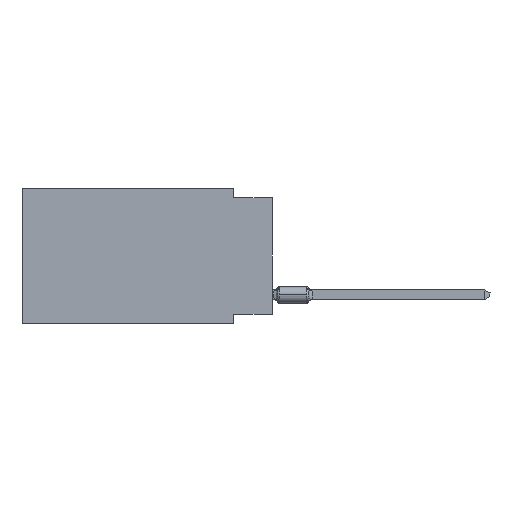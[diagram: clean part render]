
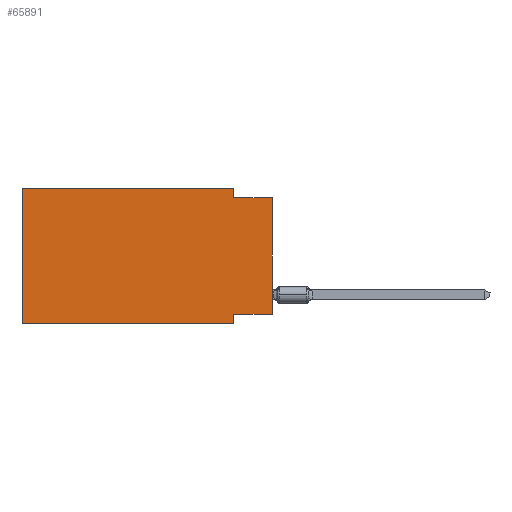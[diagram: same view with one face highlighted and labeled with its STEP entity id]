
A CAD part, left-side view. The second image highlights one B-rep face of the part: STEP entity #65891.
In plain terms, the highlighted planar face has unit normal (-1, 0, 0).
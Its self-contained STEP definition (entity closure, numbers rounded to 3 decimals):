
#831 = VECTOR ( 'NONE', #50377, 1000. ) ;
#2584 = ORIENTED_EDGE ( 'NONE', *, *, #14295, .T. ) ;
#3274 = CARTESIAN_POINT ( 'NONE',  ( 0., 2.54, -0.635 ) ) ;
#3907 = CARTESIAN_POINT ( 'NONE',  ( 0., 0., -8.255 ) ) ;
#4536 = VECTOR ( 'NONE', #19512, 1000. ) ;
#5228 = CARTESIAN_POINT ( 'NONE',  ( 0., 0., -0.635 ) ) ;
#5699 = EDGE_CURVE ( 'NONE', #62471, #52436, #19443, .T. ) ;
#6949 = LINE ( 'NONE', #36810, #34088 ) ;
#7081 = LINE ( 'NONE', #17477, #65289 ) ;
#7991 = VECTOR ( 'NONE', #15116, 1000. ) ;
#10462 = CARTESIAN_POINT ( 'NONE',  ( 0., 0., 0. ) ) ;
#11368 = LINE ( 'NONE', #37500, #57656 ) ;
#11544 = VERTEX_POINT ( 'NONE', #3907 ) ;
#14034 = VERTEX_POINT ( 'NONE', #55203 ) ;
#14129 = CARTESIAN_POINT ( 'NONE',  ( 0., 0., -0.635 ) ) ;
#14295 = EDGE_CURVE ( 'NONE', #11544, #24279, #39619, .T. ) ;
#14620 = EDGE_CURVE ( 'NONE', #14034, #16189, #7081, .T. ) ;
#15116 = DIRECTION ( 'NONE',  ( 0., -1., 0. ) ) ;
#15761 = EDGE_CURVE ( 'NONE', #16189, #62471, #41642, .T. ) ;
#16179 = DIRECTION ( 'NONE',  ( 0., -1., 0. ) ) ;
#16189 = VERTEX_POINT ( 'NONE', #53730 ) ;
#17477 = CARTESIAN_POINT ( 'NONE',  ( 0., 16.383, 0. ) ) ;
#17706 = DIRECTION ( 'NONE',  ( 0., 0., -1. ) ) ;
#19443 = LINE ( 'NONE', #45906, #58177 ) ;
#19500 = LINE ( 'NONE', #14129, #7991 ) ;
#19512 = DIRECTION ( 'NONE',  ( 0., 0., 1. ) ) ;
#19898 = CARTESIAN_POINT ( 'NONE',  ( 0., 0., -8.255 ) ) ;
#20121 = ORIENTED_EDGE ( 'NONE', *, *, #62961, .T. ) ;
#24279 = VERTEX_POINT ( 'NONE', #5228 ) ;
#27503 = CARTESIAN_POINT ( 'NONE',  ( 0., 16.383, 0. ) ) ;
#27662 = EDGE_LOOP ( 'NONE', ( #2584, #62272, #65163, #64497, #53680, #20121, #51795, #64487 ) ) ;
#29375 = VERTEX_POINT ( 'NONE', #29401 ) ;
#29401 = CARTESIAN_POINT ( 'NONE',  ( 0., 2.54, -8.89 ) ) ;
#32535 = FACE_OUTER_BOUND ( 'NONE', #27662, .T. ) ;
#33546 = DIRECTION ( 'NONE',  ( 0., 0., 1. ) ) ;
#34088 = VECTOR ( 'NONE', #56904, 1000. ) ;
#36552 = EDGE_CURVE ( 'NONE', #52436, #24279, #19500, .T. ) ;
#36810 = CARTESIAN_POINT ( 'NONE',  ( 0., 16.383, -8.89 ) ) ;
#37500 = CARTESIAN_POINT ( 'NONE',  ( 0., 2.54, -8.89 ) ) ;
#38860 = PLANE ( 'NONE',  #47267 ) ;
#39364 = LINE ( 'NONE', #19898, #831 ) ;
#39619 = LINE ( 'NONE', #10462, #4536 ) ;
#40542 = DIRECTION ( 'NONE',  ( 0., 0., -1. ) ) ;
#41642 = LINE ( 'NONE', #62106, #59028 ) ;
#45580 = CARTESIAN_POINT ( 'NONE',  ( 0., 2.54, 0. ) ) ;
#45906 = CARTESIAN_POINT ( 'NONE',  ( 0., 2.54, 0. ) ) ;
#46528 = EDGE_CURVE ( 'NONE', #11544, #56568, #39364, .T. ) ;
#47267 = AXIS2_PLACEMENT_3D ( 'NONE', #27503, #64030, #54267 ) ;
#47633 = EDGE_CURVE ( 'NONE', #56568, #29375, #11368, .T. ) ;
#50377 = DIRECTION ( 'NONE',  ( 0., 1., 0. ) ) ;
#51380 = CARTESIAN_POINT ( 'NONE',  ( 0., 2.54, -8.255 ) ) ;
#51795 = ORIENTED_EDGE ( 'NONE', *, *, #47633, .F. ) ;
#52436 = VERTEX_POINT ( 'NONE', #3274 ) ;
#53680 = ORIENTED_EDGE ( 'NONE', *, *, #14620, .F. ) ;
#53730 = CARTESIAN_POINT ( 'NONE',  ( 0., 16.383, 0. ) ) ;
#54267 = DIRECTION ( 'NONE',  ( 0., 0., -1. ) ) ;
#55203 = CARTESIAN_POINT ( 'NONE',  ( 0., 16.383, -8.89 ) ) ;
#56568 = VERTEX_POINT ( 'NONE', #51380 ) ;
#56904 = DIRECTION ( 'NONE',  ( 0., -1., 0. ) ) ;
#57656 = VECTOR ( 'NONE', #17706, 1000. ) ;
#58177 = VECTOR ( 'NONE', #40542, 1000. ) ;
#59028 = VECTOR ( 'NONE', #16179, 1000. ) ;
#62106 = CARTESIAN_POINT ( 'NONE',  ( 0., 16.383, 0. ) ) ;
#62272 = ORIENTED_EDGE ( 'NONE', *, *, #36552, .F. ) ;
#62471 = VERTEX_POINT ( 'NONE', #45580 ) ;
#62961 = EDGE_CURVE ( 'NONE', #14034, #29375, #6949, .T. ) ;
#64030 = DIRECTION ( 'NONE',  ( 1., 0., 0. ) ) ;
#64487 = ORIENTED_EDGE ( 'NONE', *, *, #46528, .F. ) ;
#64497 = ORIENTED_EDGE ( 'NONE', *, *, #15761, .F. ) ;
#65163 = ORIENTED_EDGE ( 'NONE', *, *, #5699, .F. ) ;
#65289 = VECTOR ( 'NONE', #33546, 1000. ) ;
#65891 = ADVANCED_FACE ( 'NONE', ( #32535 ), #38860, .F. ) ;
